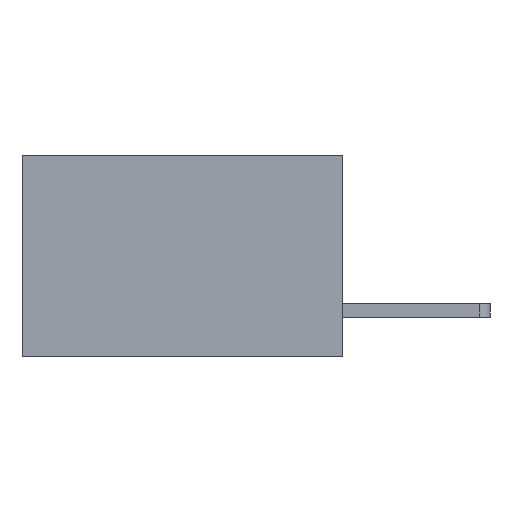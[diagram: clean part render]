
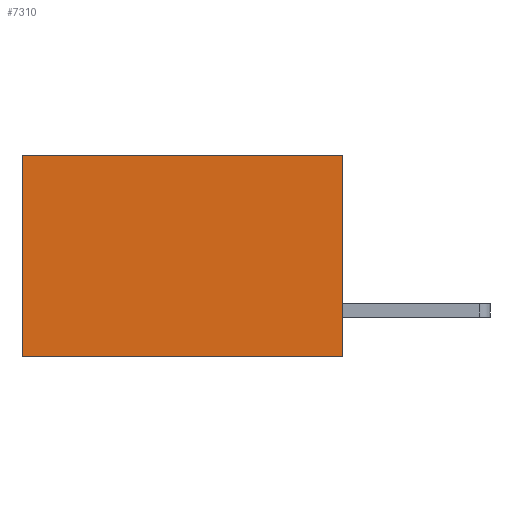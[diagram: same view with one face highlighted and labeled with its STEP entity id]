
A CAD part, left-side view. The second image highlights one B-rep face of the part: STEP entity #7310.
In plain terms, the highlighted planar face has unit normal (-1, 0, 0).
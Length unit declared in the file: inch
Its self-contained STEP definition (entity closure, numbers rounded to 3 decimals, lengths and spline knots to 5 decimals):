
#227 = LINE ( 'NONE', #4352, #3418 ) ;
#380 = EDGE_CURVE ( 'NONE', #5975, #3234, #227, .T. ) ;
#701 = DIRECTION ( 'NONE',  ( 0., 0., -1. ) ) ;
#704 = DIRECTION ( 'NONE',  ( 1., 0., 0. ) ) ;
#712 = CARTESIAN_POINT ( 'NONE',  ( 0.277, 0., -0.37 ) ) ;
#721 = PLANE ( 'NONE',  #6596 ) ;
#851 = VERTEX_POINT ( 'NONE', #2611 ) ;
#859 = ORIENTED_EDGE ( 'NONE', *, *, #380, .T. ) ;
#1270 = VECTOR ( 'NONE', #5789, 39.37008 ) ;
#1672 = VECTOR ( 'NONE', #6699, 39.37008 ) ;
#2100 = ORIENTED_EDGE ( 'NONE', *, *, #4211, .T. ) ;
#2199 = CARTESIAN_POINT ( 'NONE',  ( 0.277, 0.59, 0. ) ) ;
#2611 = CARTESIAN_POINT ( 'NONE',  ( 0.277, 0.59, -0.37 ) ) ;
#2681 = DIRECTION ( 'NONE',  ( 0., 1., 0. ) ) ;
#3234 = VERTEX_POINT ( 'NONE', #2199 ) ;
#3407 = LINE ( 'NONE', #6438, #1672 ) ;
#3418 = VECTOR ( 'NONE', #2681, 39.37008 ) ;
#3580 = EDGE_CURVE ( 'NONE', #5975, #6703, #3407, .T. ) ;
#3864 = ORIENTED_EDGE ( 'NONE', *, *, #5497, .F. ) ;
#4211 = EDGE_CURVE ( 'NONE', #3234, #851, #5373, .T. ) ;
#4352 = CARTESIAN_POINT ( 'NONE',  ( 0.277, 0., 0. ) ) ;
#4810 = CARTESIAN_POINT ( 'NONE',  ( 0.277, 0.59, -0.37 ) ) ;
#4831 = DIRECTION ( 'NONE',  ( 0., 0., -1. ) ) ;
#5108 = CARTESIAN_POINT ( 'NONE',  ( 0.277, 0., -0.37 ) ) ;
#5162 = VECTOR ( 'NONE', #4831, 39.37008 ) ;
#5373 = LINE ( 'NONE', #4810, #5162 ) ;
#5497 = EDGE_CURVE ( 'NONE', #6703, #851, #6096, .T. ) ;
#5540 = EDGE_LOOP ( 'NONE', ( #2100, #3864, #6978, #859 ) ) ;
#5577 = CARTESIAN_POINT ( 'NONE',  ( 0.277, 0., -0.37 ) ) ;
#5789 = DIRECTION ( 'NONE',  ( 0., 1., 0. ) ) ;
#5975 = VERTEX_POINT ( 'NONE', #7536 ) ;
#6096 = LINE ( 'NONE', #5577, #1270 ) ;
#6438 = CARTESIAN_POINT ( 'NONE',  ( 0.277, 0., -0.37 ) ) ;
#6596 = AXIS2_PLACEMENT_3D ( 'NONE', #712, #704, #701 ) ;
#6699 = DIRECTION ( 'NONE',  ( 0., 0., -1. ) ) ;
#6703 = VERTEX_POINT ( 'NONE', #5108 ) ;
#6978 = ORIENTED_EDGE ( 'NONE', *, *, #3580, .F. ) ;
#7040 = FACE_OUTER_BOUND ( 'NONE', #5540, .T. ) ;
#7310 = ADVANCED_FACE ( 'NONE', ( #7040 ), #721, .F. ) ;
#7536 = CARTESIAN_POINT ( 'NONE',  ( 0.277, 0., 0. ) ) ;
